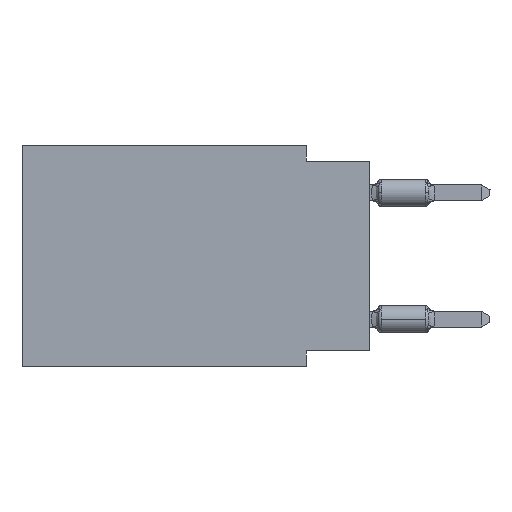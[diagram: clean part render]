
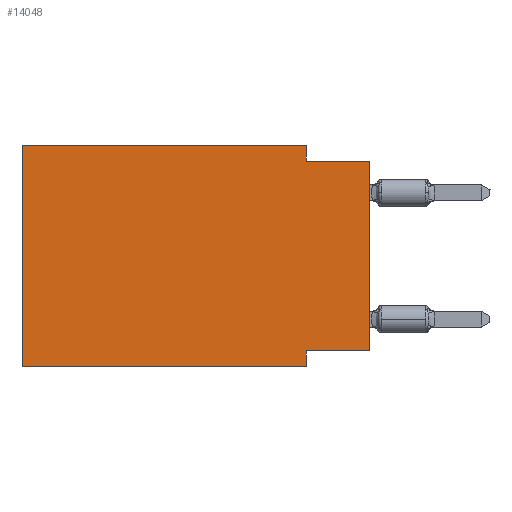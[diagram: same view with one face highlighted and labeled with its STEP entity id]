
A CAD part, left-side view. The second image highlights one B-rep face of the part: STEP entity #14048.
In plain terms, the highlighted planar face has unit normal (-1, 0, 0).
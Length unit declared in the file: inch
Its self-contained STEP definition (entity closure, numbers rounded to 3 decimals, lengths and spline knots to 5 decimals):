
#596 = EDGE_CURVE ( 'NONE', #10018, #23646, #26404, .T. ) ;
#733 = EDGE_CURVE ( 'NONE', #10018, #27618, #30746, .T. ) ;
#987 = ORIENTED_EDGE ( 'NONE', *, *, #596, .F. ) ;
#1307 = DIRECTION ( 'NONE',  ( 0., 0., -1. ) ) ;
#2437 = DIRECTION ( 'NONE',  ( 0., 0., -1. ) ) ;
#2852 = ORIENTED_EDGE ( 'NONE', *, *, #8097, .F. ) ;
#2862 = VECTOR ( 'NONE', #4034, 39.37008 ) ;
#3066 = DIRECTION ( 'NONE',  ( 0., 0., -1. ) ) ;
#3884 = VERTEX_POINT ( 'NONE', #10939 ) ;
#4034 = DIRECTION ( 'NONE',  ( 0., -1., 0. ) ) ;
#4416 = EDGE_LOOP ( 'NONE', ( #15553, #24846, #2852, #18620, #11785, #10094, #31527, #987 ) ) ;
#4650 = FACE_OUTER_BOUND ( 'NONE', #4416, .T. ) ;
#6356 = DIRECTION ( 'NONE',  ( 0., 1., 0. ) ) ;
#6566 = LINE ( 'NONE', #6743, #2862 ) ;
#6605 = CARTESIAN_POINT ( 'NONE',  ( 0., 0.55, 0. ) ) ;
#6743 = CARTESIAN_POINT ( 'NONE',  ( 0., 0.55, 0. ) ) ;
#7826 = VERTEX_POINT ( 'NONE', #20620 ) ;
#8097 = EDGE_CURVE ( 'NONE', #32348, #7826, #17858, .T. ) ;
#8160 = PLANE ( 'NONE',  #24409 ) ;
#8415 = VECTOR ( 'NONE', #1307, 39.37008 ) ;
#8715 = CARTESIAN_POINT ( 'NONE',  ( 0., 0.55, -0.35 ) ) ;
#8977 = CARTESIAN_POINT ( 'NONE',  ( 0., 0.1, 0. ) ) ;
#9111 = VECTOR ( 'NONE', #2437, 39.37008 ) ;
#9254 = VECTOR ( 'NONE', #22210, 39.37008 ) ;
#10018 = VERTEX_POINT ( 'NONE', #32399 ) ;
#10094 = ORIENTED_EDGE ( 'NONE', *, *, #16992, .T. ) ;
#10634 = CARTESIAN_POINT ( 'NONE',  ( 0., 0.55, -0.35 ) ) ;
#10721 = DIRECTION ( 'NONE',  ( 0., 0., 1. ) ) ;
#10939 = CARTESIAN_POINT ( 'NONE',  ( 0., 0.1, -0.35 ) ) ;
#11785 = ORIENTED_EDGE ( 'NONE', *, *, #16292, .F. ) ;
#11839 = CARTESIAN_POINT ( 'NONE',  ( 0., 0., -0.025 ) ) ;
#13510 = CARTESIAN_POINT ( 'NONE',  ( 0., 0., -0.325 ) ) ;
#14048 = ADVANCED_FACE ( 'NONE', ( #4650 ), #8160, .F. ) ;
#14281 = EDGE_CURVE ( 'NONE', #7826, #27618, #24927, .T. ) ;
#14393 = CARTESIAN_POINT ( 'NONE',  ( 0., 0.1, -0.325 ) ) ;
#15553 = ORIENTED_EDGE ( 'NONE', *, *, #733, .T. ) ;
#16292 = EDGE_CURVE ( 'NONE', #26639, #21878, #24606, .T. ) ;
#16992 = EDGE_CURVE ( 'NONE', #26639, #3884, #29732, .T. ) ;
#17858 = LINE ( 'NONE', #32812, #9111 ) ;
#17956 = EDGE_CURVE ( 'NONE', #21878, #32348, #6566, .T. ) ;
#18338 = CARTESIAN_POINT ( 'NONE',  ( 0., 0.55, 0. ) ) ;
#18620 = ORIENTED_EDGE ( 'NONE', *, *, #17956, .F. ) ;
#20010 = DIRECTION ( 'NONE',  ( 0., 0., 1. ) ) ;
#20620 = CARTESIAN_POINT ( 'NONE',  ( 0., 0.1, -0.025 ) ) ;
#20885 = DIRECTION ( 'NONE',  ( 1., 0., 0. ) ) ;
#20928 = EDGE_CURVE ( 'NONE', #23646, #3884, #32201, .T. ) ;
#20973 = DIRECTION ( 'NONE',  ( 0., -1., 0. ) ) ;
#21878 = VERTEX_POINT ( 'NONE', #25961 ) ;
#22210 = DIRECTION ( 'NONE',  ( 0., -1., 0. ) ) ;
#22527 = CARTESIAN_POINT ( 'NONE',  ( 0., 0.1, -0.35 ) ) ;
#23409 = VECTOR ( 'NONE', #20973, 39.37008 ) ;
#23646 = VERTEX_POINT ( 'NONE', #14393 ) ;
#24409 = AXIS2_PLACEMENT_3D ( 'NONE', #18338, #20885, #3066 ) ;
#24606 = LINE ( 'NONE', #6605, #25607 ) ;
#24846 = ORIENTED_EDGE ( 'NONE', *, *, #14281, .F. ) ;
#24927 = LINE ( 'NONE', #32911, #9254 ) ;
#25496 = CARTESIAN_POINT ( 'NONE',  ( 0., 0., 0. ) ) ;
#25607 = VECTOR ( 'NONE', #20010, 39.37008 ) ;
#25961 = CARTESIAN_POINT ( 'NONE',  ( 0., 0.55, 0. ) ) ;
#26404 = LINE ( 'NONE', #13510, #27600 ) ;
#26639 = VERTEX_POINT ( 'NONE', #8715 ) ;
#27600 = VECTOR ( 'NONE', #6356, 39.37008 ) ;
#27618 = VERTEX_POINT ( 'NONE', #11839 ) ;
#29732 = LINE ( 'NONE', #10634, #23409 ) ;
#29760 = VECTOR ( 'NONE', #10721, 39.37008 ) ;
#30746 = LINE ( 'NONE', #25496, #29760 ) ;
#31527 = ORIENTED_EDGE ( 'NONE', *, *, #20928, .F. ) ;
#32201 = LINE ( 'NONE', #22527, #8415 ) ;
#32348 = VERTEX_POINT ( 'NONE', #8977 ) ;
#32399 = CARTESIAN_POINT ( 'NONE',  ( 0., 0., -0.325 ) ) ;
#32812 = CARTESIAN_POINT ( 'NONE',  ( 0., 0.1, 0. ) ) ;
#32911 = CARTESIAN_POINT ( 'NONE',  ( 0., 0., -0.025 ) ) ;
